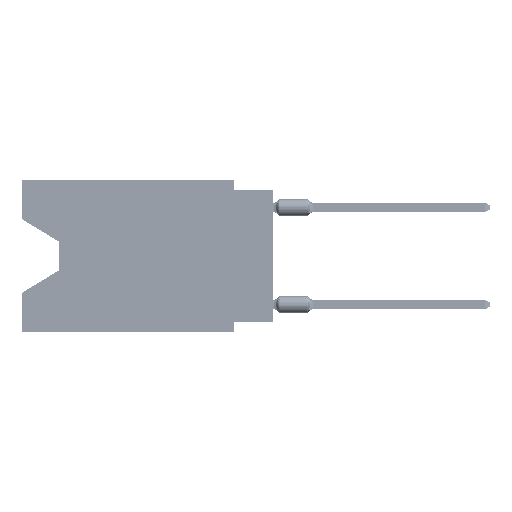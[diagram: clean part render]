
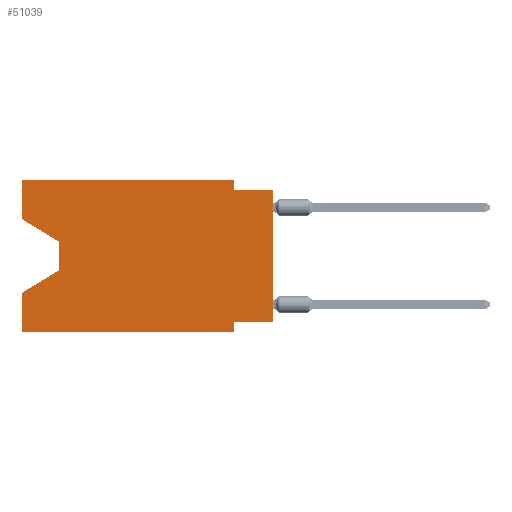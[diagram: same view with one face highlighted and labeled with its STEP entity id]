
A CAD part, left-side view. The second image highlights one B-rep face of the part: STEP entity #51039.
In plain terms, the highlighted planar face has unit normal (-1, 0, 0).
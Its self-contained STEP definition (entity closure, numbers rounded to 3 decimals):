
#828 = CARTESIAN_POINT ( 'NONE',  ( 0., 16.383, 0. ) ) ;
#1775 = CARTESIAN_POINT ( 'NONE',  ( 0., 16.383, -9.906 ) ) ;
#3680 = ORIENTED_EDGE ( 'NONE', *, *, #81469, .T. ) ;
#5832 = VECTOR ( 'NONE', #24931, 1000. ) ;
#6849 = CARTESIAN_POINT ( 'NONE',  ( 0., 13.97, -5.893 ) ) ;
#7890 = CARTESIAN_POINT ( 'NONE',  ( 0., 2.54, -0.635 ) ) ;
#8220 = VECTOR ( 'NONE', #20076, 1000. ) ;
#8390 = CARTESIAN_POINT ( 'NONE',  ( 0., 2.54, -9.271 ) ) ;
#9062 = LINE ( 'NONE', #1775, #79748 ) ;
#9557 = EDGE_CURVE ( 'NONE', #88120, #81093, #57194, .T. ) ;
#9714 = CARTESIAN_POINT ( 'NONE',  ( 0., 0., -0.635 ) ) ;
#10831 = ORIENTED_EDGE ( 'NONE', *, *, #48278, .F. ) ;
#11622 = CARTESIAN_POINT ( 'NONE',  ( 0., 13.97, -4.013 ) ) ;
#12353 = EDGE_CURVE ( 'NONE', #81093, #54999, #60184, .T. ) ;
#12676 = DIRECTION ( 'NONE',  ( 0., 0., 1. ) ) ;
#13983 = ORIENTED_EDGE ( 'NONE', *, *, #42183, .F. ) ;
#14750 = VERTEX_POINT ( 'NONE', #8390 ) ;
#16562 = ORIENTED_EDGE ( 'NONE', *, *, #46712, .F. ) ;
#16751 = CARTESIAN_POINT ( 'NONE',  ( 0., 2.54, -9.906 ) ) ;
#16904 = EDGE_CURVE ( 'NONE', #33179, #22523, #52790, .T. ) ;
#16953 = CARTESIAN_POINT ( 'NONE',  ( 0., 0., -0.635 ) ) ;
#18137 = EDGE_LOOP ( 'NONE', ( #59040, #24275, #68812, #10831, #68739, #65100, #13983, #3680, #22653, #87166, #51483, #16562 ) ) ;
#18623 = DIRECTION ( 'NONE',  ( 0., 1., 0. ) ) ;
#19633 = CARTESIAN_POINT ( 'NONE',  ( 0., 13.97, -5.893 ) ) ;
#20076 = DIRECTION ( 'NONE',  ( 0., 0.855, -0.519 ) ) ;
#21887 = CARTESIAN_POINT ( 'NONE',  ( 0., 0., -9.271 ) ) ;
#22240 = DIRECTION ( 'NONE',  ( 1., 0., 0. ) ) ;
#22523 = VERTEX_POINT ( 'NONE', #7890 ) ;
#22653 = ORIENTED_EDGE ( 'NONE', *, *, #77691, .F. ) ;
#23793 = DIRECTION ( 'NONE',  ( 0., -1., 0. ) ) ;
#24275 = ORIENTED_EDGE ( 'NONE', *, *, #9557, .T. ) ;
#24360 = VERTEX_POINT ( 'NONE', #25443 ) ;
#24931 = DIRECTION ( 'NONE',  ( 0., 0., -1. ) ) ;
#25088 = DIRECTION ( 'NONE',  ( 0., 0., 1. ) ) ;
#25380 = VERTEX_POINT ( 'NONE', #21887 ) ;
#25443 = CARTESIAN_POINT ( 'NONE',  ( 0., 16.383, -9.906 ) ) ;
#25657 = VECTOR ( 'NONE', #18623, 1000. ) ;
#26793 = LINE ( 'NONE', #76006, #53961 ) ;
#27265 = FACE_OUTER_BOUND ( 'NONE', #18137, .T. ) ;
#27742 = VECTOR ( 'NONE', #80312, 1000. ) ;
#31846 = DIRECTION ( 'NONE',  ( 0., 0., -1. ) ) ;
#31991 = LINE ( 'NONE', #33817, #27742 ) ;
#32032 = VECTOR ( 'NONE', #45677, 1000. ) ;
#32388 = LINE ( 'NONE', #80684, #81678 ) ;
#32817 = VERTEX_POINT ( 'NONE', #73980 ) ;
#33179 = VERTEX_POINT ( 'NONE', #73422 ) ;
#33360 = VERTEX_POINT ( 'NONE', #61998 ) ;
#33817 = CARTESIAN_POINT ( 'NONE',  ( 0., 16.383, -2.546 ) ) ;
#34437 = DIRECTION ( 'NONE',  ( 0., 0., -1. ) ) ;
#35010 = DIRECTION ( 'NONE',  ( 0., 0., -1. ) ) ;
#37812 = EDGE_CURVE ( 'NONE', #32817, #88120, #31991, .T. ) ;
#38656 = CARTESIAN_POINT ( 'NONE',  ( 0., 0., -9.271 ) ) ;
#41861 = DIRECTION ( 'NONE',  ( 0., -1., 0. ) ) ;
#41959 = EDGE_CURVE ( 'NONE', #86101, #33179, #62894, .T. ) ;
#42153 = CARTESIAN_POINT ( 'NONE',  ( 0., 13.97, -4.013 ) ) ;
#42183 = EDGE_CURVE ( 'NONE', #25380, #14750, #58300, .T. ) ;
#43871 = LINE ( 'NONE', #16953, #76735 ) ;
#45102 = VERTEX_POINT ( 'NONE', #9714 ) ;
#45313 = CARTESIAN_POINT ( 'NONE',  ( 0., 16.383, -7.36 ) ) ;
#45545 = VECTOR ( 'NONE', #46976, 1000. ) ;
#45677 = DIRECTION ( 'NONE',  ( 0., 0., 1. ) ) ;
#46712 = EDGE_CURVE ( 'NONE', #32817, #86101, #60247, .T. ) ;
#46976 = DIRECTION ( 'NONE',  ( 0., -1., 0. ) ) ;
#48278 = EDGE_CURVE ( 'NONE', #24360, #54999, #32388, .T. ) ;
#51039 = ADVANCED_FACE ( 'NONE', ( #27265 ), #76470, .F. ) ;
#51463 = CARTESIAN_POINT ( 'NONE',  ( 0., 2.54, 0. ) ) ;
#51483 = ORIENTED_EDGE ( 'NONE', *, *, #41959, .F. ) ;
#52273 = EDGE_CURVE ( 'NONE', #14750, #33360, #86470, .T. ) ;
#52790 = LINE ( 'NONE', #51463, #89388 ) ;
#53793 = CARTESIAN_POINT ( 'NONE',  ( 0., 16.383, 0. ) ) ;
#53961 = VECTOR ( 'NONE', #12676, 1000. ) ;
#54999 = VERTEX_POINT ( 'NONE', #45313 ) ;
#57194 = LINE ( 'NONE', #42153, #85089 ) ;
#58300 = LINE ( 'NONE', #38656, #25657 ) ;
#59040 = ORIENTED_EDGE ( 'NONE', *, *, #37812, .T. ) ;
#60184 = LINE ( 'NONE', #19633, #8220 ) ;
#60247 = LINE ( 'NONE', #73053, #32032 ) ;
#61998 = CARTESIAN_POINT ( 'NONE',  ( 0., 2.54, -9.906 ) ) ;
#62894 = LINE ( 'NONE', #53793, #45545 ) ;
#65100 = ORIENTED_EDGE ( 'NONE', *, *, #52273, .F. ) ;
#68739 = ORIENTED_EDGE ( 'NONE', *, *, #86074, .T. ) ;
#68812 = ORIENTED_EDGE ( 'NONE', *, *, #12353, .T. ) ;
#73053 = CARTESIAN_POINT ( 'NONE',  ( 0., 16.383, 0. ) ) ;
#73422 = CARTESIAN_POINT ( 'NONE',  ( 0., 2.54, 0. ) ) ;
#73980 = CARTESIAN_POINT ( 'NONE',  ( 0., 16.383, -2.546 ) ) ;
#76006 = CARTESIAN_POINT ( 'NONE',  ( 0., 0., 0. ) ) ;
#76470 = PLANE ( 'NONE',  #82854 ) ;
#76735 = VECTOR ( 'NONE', #23793, 1000. ) ;
#77419 = CARTESIAN_POINT ( 'NONE',  ( 0., 16.383, 0. ) ) ;
#77691 = EDGE_CURVE ( 'NONE', #22523, #45102, #43871, .T. ) ;
#79748 = VECTOR ( 'NONE', #41861, 1000. ) ;
#80312 = DIRECTION ( 'NONE',  ( 0., -0.855, -0.519 ) ) ;
#80684 = CARTESIAN_POINT ( 'NONE',  ( 0., 16.383, 0. ) ) ;
#81093 = VERTEX_POINT ( 'NONE', #6849 ) ;
#81469 = EDGE_CURVE ( 'NONE', #25380, #45102, #26793, .T. ) ;
#81678 = VECTOR ( 'NONE', #25088, 1000. ) ;
#82854 = AXIS2_PLACEMENT_3D ( 'NONE', #828, #22240, #35010 ) ;
#85089 = VECTOR ( 'NONE', #34437, 1000. ) ;
#86074 = EDGE_CURVE ( 'NONE', #24360, #33360, #9062, .T. ) ;
#86101 = VERTEX_POINT ( 'NONE', #77419 ) ;
#86470 = LINE ( 'NONE', #16751, #5832 ) ;
#87166 = ORIENTED_EDGE ( 'NONE', *, *, #16904, .F. ) ;
#88120 = VERTEX_POINT ( 'NONE', #11622 ) ;
#89388 = VECTOR ( 'NONE', #31846, 1000. ) ;
